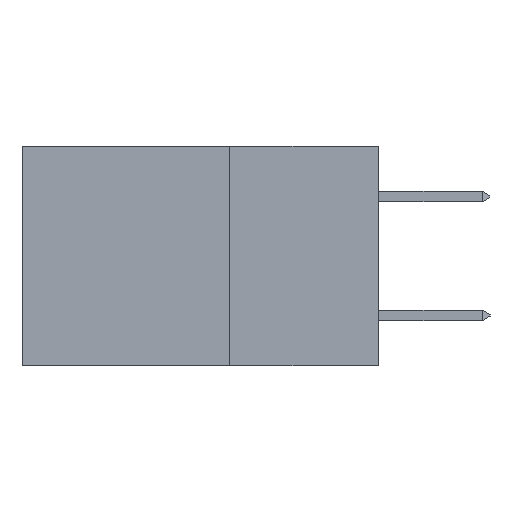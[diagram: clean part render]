
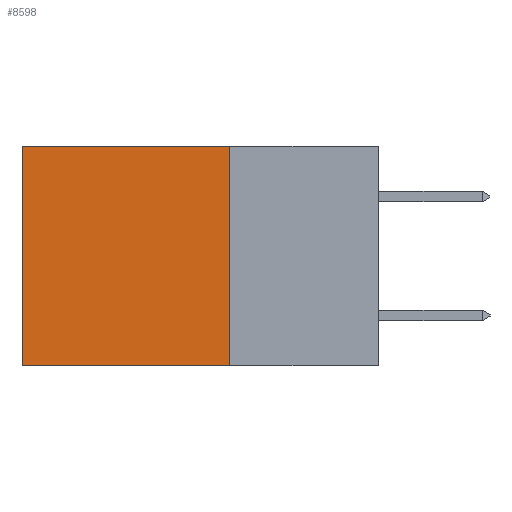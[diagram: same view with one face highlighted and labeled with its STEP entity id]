
A CAD part, left-side view. The second image highlights one B-rep face of the part: STEP entity #8598.
In plain terms, the highlighted planar face has unit normal (-1, 0, 0).
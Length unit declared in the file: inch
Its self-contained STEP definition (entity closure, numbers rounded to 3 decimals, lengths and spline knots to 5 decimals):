
#126 = CARTESIAN_POINT ( 'NONE',  ( 0.2615, 0.6, 0. ) ) ;
#308 = CARTESIAN_POINT ( 'NONE',  ( 0.2615, 0.25, -0.37 ) ) ;
#447 = LINE ( 'NONE', #4137, #6801 ) ;
#468 = DIRECTION ( 'NONE',  ( 0., 0., -1. ) ) ;
#1095 = VERTEX_POINT ( 'NONE', #11917 ) ;
#1348 = ORIENTED_EDGE ( 'NONE', *, *, #12541, .F. ) ;
#2964 = AXIS2_PLACEMENT_3D ( 'NONE', #10027, #10016, #9997 ) ;
#3426 = VECTOR ( 'NONE', #7628, 39.37008 ) ;
#3901 = VERTEX_POINT ( 'NONE', #126 ) ;
#4087 = DIRECTION ( 'NONE',  ( 0., 1., 0. ) ) ;
#4137 = CARTESIAN_POINT ( 'NONE',  ( 0.2615, 0.25, 0. ) ) ;
#4842 = ORIENTED_EDGE ( 'NONE', *, *, #7554, .T. ) ;
#4936 = LINE ( 'NONE', #10723, #8236 ) ;
#5908 = EDGE_CURVE ( 'NONE', #11735, #1095, #11407, .T. ) ;
#6721 = ORIENTED_EDGE ( 'NONE', *, *, #8922, .T. ) ;
#6801 = VECTOR ( 'NONE', #4087, 39.37008 ) ;
#7130 = LINE ( 'NONE', #7728, #3426 ) ;
#7248 = VERTEX_POINT ( 'NONE', #10032 ) ;
#7554 = EDGE_CURVE ( 'NONE', #11735, #3901, #447, .T. ) ;
#7628 = DIRECTION ( 'NONE',  ( 0., 0., -1. ) ) ;
#7728 = CARTESIAN_POINT ( 'NONE',  ( 0.2615, 0.6, -0.37 ) ) ;
#8236 = VECTOR ( 'NONE', #11882, 39.37008 ) ;
#8509 = EDGE_LOOP ( 'NONE', ( #6721, #1348, #13461, #4842 ) ) ;
#8598 = ADVANCED_FACE ( 'NONE', ( #11324 ), #10192, .F. ) ;
#8920 = CARTESIAN_POINT ( 'NONE',  ( 0.2615, 0.25, 0. ) ) ;
#8922 = EDGE_CURVE ( 'NONE', #3901, #7248, #7130, .T. ) ;
#9997 = DIRECTION ( 'NONE',  ( 0., 0., -1. ) ) ;
#10016 = DIRECTION ( 'NONE',  ( 1., 0., 0. ) ) ;
#10027 = CARTESIAN_POINT ( 'NONE',  ( 0.2615, 0.25, -0.37 ) ) ;
#10032 = CARTESIAN_POINT ( 'NONE',  ( 0.2615, 0.6, -0.37 ) ) ;
#10192 = PLANE ( 'NONE',  #2964 ) ;
#10723 = CARTESIAN_POINT ( 'NONE',  ( 0.2615, 0.25, -0.37 ) ) ;
#11324 = FACE_OUTER_BOUND ( 'NONE', #8509, .T. ) ;
#11407 = LINE ( 'NONE', #308, #14558 ) ;
#11735 = VERTEX_POINT ( 'NONE', #8920 ) ;
#11882 = DIRECTION ( 'NONE',  ( 0., 1., 0. ) ) ;
#11917 = CARTESIAN_POINT ( 'NONE',  ( 0.2615, 0.25, -0.37 ) ) ;
#12541 = EDGE_CURVE ( 'NONE', #1095, #7248, #4936, .T. ) ;
#13461 = ORIENTED_EDGE ( 'NONE', *, *, #5908, .F. ) ;
#14558 = VECTOR ( 'NONE', #468, 39.37008 ) ;
